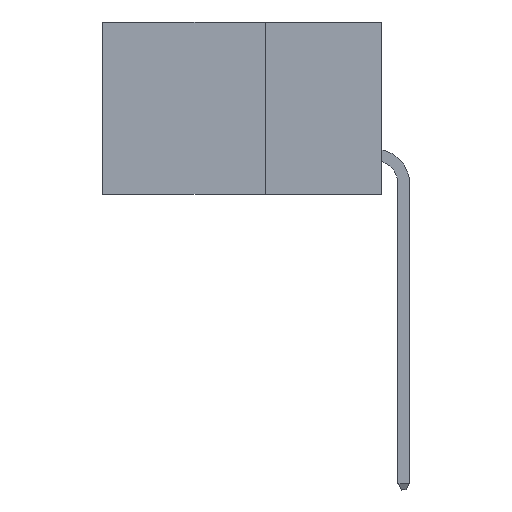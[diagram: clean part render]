
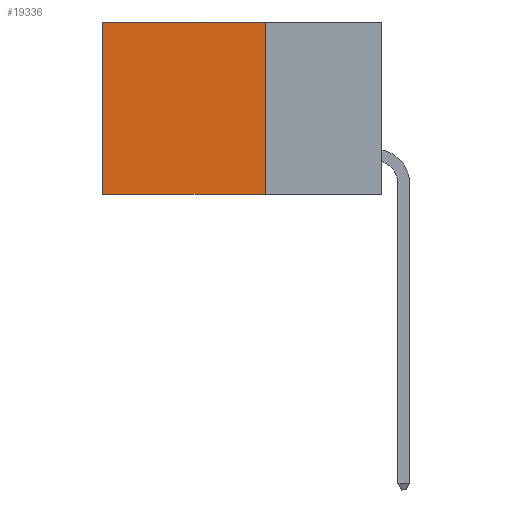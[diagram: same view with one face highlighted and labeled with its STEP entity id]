
A CAD part, left-side view. The second image highlights one B-rep face of the part: STEP entity #19336.
In plain terms, the highlighted planar face has unit normal (-1, 0, 0).
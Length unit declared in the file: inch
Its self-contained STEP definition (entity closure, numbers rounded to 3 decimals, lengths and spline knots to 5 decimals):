
#377 = VECTOR ( 'NONE', #3157, 39.37008 ) ;
#1137 = ORIENTED_EDGE ( 'NONE', *, *, #14053, .T. ) ;
#2206 = AXIS2_PLACEMENT_3D ( 'NONE', #7689, #13529, #5856 ) ;
#2743 = VERTEX_POINT ( 'NONE', #8811 ) ;
#2810 = ORIENTED_EDGE ( 'NONE', *, *, #17444, .F. ) ;
#3071 = PLANE ( 'NONE',  #2206 ) ;
#3108 = VECTOR ( 'NONE', #7350, 39.37008 ) ;
#3157 = DIRECTION ( 'NONE',  ( 0., 1., 0. ) ) ;
#4342 = EDGE_CURVE ( 'NONE', #19896, #2743, #16308, .T. ) ;
#5704 = VECTOR ( 'NONE', #12700, 39.37008 ) ;
#5763 = CARTESIAN_POINT ( 'NONE',  ( 0.2875, 0.25, 0. ) ) ;
#5856 = DIRECTION ( 'NONE',  ( 0., 0., -1. ) ) ;
#6141 = CARTESIAN_POINT ( 'NONE',  ( 0.2875, 0.25, 0. ) ) ;
#6142 = CARTESIAN_POINT ( 'NONE',  ( 0.2875, 0.6, 0. ) ) ;
#7350 = DIRECTION ( 'NONE',  ( 0., 0., -1. ) ) ;
#7689 = CARTESIAN_POINT ( 'NONE',  ( 0.2875, 0.25, 0. ) ) ;
#7862 = CARTESIAN_POINT ( 'NONE',  ( 0.2875, 0.25, -0.37 ) ) ;
#8811 = CARTESIAN_POINT ( 'NONE',  ( 0.2875, 0.6, -0.37 ) ) ;
#10062 = ORIENTED_EDGE ( 'NONE', *, *, #4342, .T. ) ;
#10139 = VERTEX_POINT ( 'NONE', #5763 ) ;
#10232 = FACE_OUTER_BOUND ( 'NONE', #11746, .T. ) ;
#10680 = CARTESIAN_POINT ( 'NONE',  ( 0.2875, 0.6, 0. ) ) ;
#10769 = LINE ( 'NONE', #7862, #5704 ) ;
#10979 = VECTOR ( 'NONE', #12291, 39.37008 ) ;
#11419 = LINE ( 'NONE', #6141, #377 ) ;
#11746 = EDGE_LOOP ( 'NONE', ( #10062, #2810, #15388, #1137 ) ) ;
#11855 = CARTESIAN_POINT ( 'NONE',  ( 0.2875, 0.25, 0. ) ) ;
#12291 = DIRECTION ( 'NONE',  ( 0., 0., -1. ) ) ;
#12700 = DIRECTION ( 'NONE',  ( 0., 1., 0. ) ) ;
#12950 = LINE ( 'NONE', #11855, #3108 ) ;
#13529 = DIRECTION ( 'NONE',  ( 1., 0., 0. ) ) ;
#14053 = EDGE_CURVE ( 'NONE', #10139, #19896, #11419, .T. ) ;
#14757 = CARTESIAN_POINT ( 'NONE',  ( 0.2875, 0.25, -0.37 ) ) ;
#15388 = ORIENTED_EDGE ( 'NONE', *, *, #17361, .F. ) ;
#16308 = LINE ( 'NONE', #6142, #10979 ) ;
#17361 = EDGE_CURVE ( 'NONE', #10139, #19674, #12950, .T. ) ;
#17444 = EDGE_CURVE ( 'NONE', #19674, #2743, #10769, .T. ) ;
#19336 = ADVANCED_FACE ( 'NONE', ( #10232 ), #3071, .F. ) ;
#19674 = VERTEX_POINT ( 'NONE', #14757 ) ;
#19896 = VERTEX_POINT ( 'NONE', #10680 ) ;
